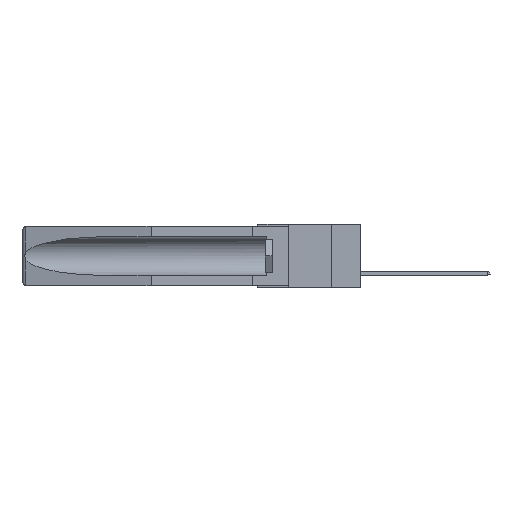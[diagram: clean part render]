
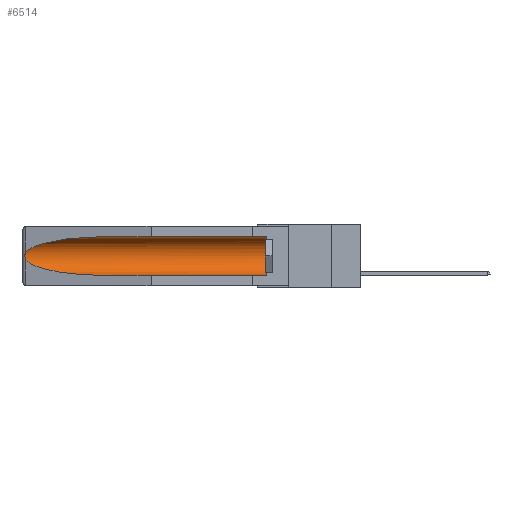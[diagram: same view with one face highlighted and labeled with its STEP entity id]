
A CAD part, left-side view. The second image highlights one B-rep face of the part: STEP entity #6514.
In plain terms, the highlighted cylindrical face has radius 2.857 mm (diameter 5.715 mm), a partial arc.
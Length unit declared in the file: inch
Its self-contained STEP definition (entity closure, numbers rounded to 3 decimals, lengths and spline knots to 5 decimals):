
#280 = CARTESIAN_POINT ( 'NONE',  ( 0.155, -0.30754, -0.1715 ) ) ;
#598 = CARTESIAN_POINT ( 'NONE',  ( 0.26537, 1.52718, -0.14972 ) ) ;
#786 = CARTESIAN_POINT ( 'NONE',  ( 0.155, 1.07973, -0.059 ) ) ;
#916 = ORIENTED_EDGE ( 'NONE', *, *, #7223, .T. ) ;
#985 = VERTEX_POINT ( 'NONE', #13216 ) ;
#1400 = VERTEX_POINT ( 'NONE', #3922 ) ;
#1910 = EDGE_CURVE ( 'NONE', #15032, #1400, #6840, .T. ) ;
#2029 = CARTESIAN_POINT ( 'NONE',  ( 0.2673, 1.5327, -0.16383 ) ) ;
#2625 = CARTESIAN_POINT ( 'NONE',  ( 0.155, 1.07973, -0.059 ) ) ;
#3262 = CARTESIAN_POINT ( 'NONE',  ( 0.26537, 1.52718, -0.19328 ) ) ;
#3442 = CARTESIAN_POINT ( 'NONE',  ( 0.26597, 1.52961, -0.15275 ) ) ;
#3922 = CARTESIAN_POINT ( 'NONE',  ( 0.26537, 1.52718, -0.19328 ) ) ;
#4167 = EDGE_CURVE ( 'NONE', #17128, #8973, #11744, .T. ) ;
#5041 = CARTESIAN_POINT ( 'NONE',  ( 0.155, 0.126, -0.284 ) ) ;
#5100 = EDGE_LOOP ( 'NONE', ( #5375, #6243, #15499, #18065, #916, #15361 ) ) ;
#5111 = EDGE_CURVE ( 'NONE', #8973, #15032, #5616, .T. ) ;
#5375 = ORIENTED_EDGE ( 'NONE', *, *, #5111, .T. ) ;
#5616 =( BOUNDED_CURVE ( )  B_SPLINE_CURVE ( 3, ( #786, #11089, #15373, #16802 ),
 .UNSPECIFIED., .F., .F. ) 
 B_SPLINE_CURVE_WITH_KNOTS ( ( 4, 4 ),
 ( 4.71239, 6.08839 ),
 .UNSPECIFIED. ) 
 CURVE ( )  GEOMETRIC_REPRESENTATION_ITEM ( )  RATIONAL_B_SPLINE_CURVE ( ( 1., 0.848, 0.848, 1. ) ) 
 REPRESENTATION_ITEM ( '' )  );
#6062 = DIRECTION ( 'NONE',  ( 0., 0., 1. ) ) ;
#6236 =( BOUNDED_CURVE ( )  B_SPLINE_CURVE ( 3, ( #3262, #13537, #9177, #13908 ),
 .UNSPECIFIED., .F., .F. ) 
 B_SPLINE_CURVE_WITH_KNOTS ( ( 4, 4 ),
 ( 0.1948, 1.5708 ),
 .UNSPECIFIED. ) 
 CURVE ( )  GEOMETRIC_REPRESENTATION_ITEM ( )  RATIONAL_B_SPLINE_CURVE ( ( 1., 0.848, 0.848, 1. ) ) 
 REPRESENTATION_ITEM ( '' )  );
#6243 = ORIENTED_EDGE ( 'NONE', *, *, #1910, .T. ) ;
#6263 = VERTEX_POINT ( 'NONE', #5041 ) ;
#6514 = ADVANCED_FACE ( 'NONE', ( #8643 ), #11636, .F. ) ;
#6644 = CARTESIAN_POINT ( 'NONE',  ( 0.26597, 1.5296, -0.19026 ) ) ;
#6840 = B_SPLINE_CURVE_WITH_KNOTS ( 'NONE', 3,
 ( #598, #3442, #9364, #2029, #12302, #13774, #10901, #18481, #6644, #12610 ),
 .UNSPECIFIED., .F., .F.,
 ( 4, 2, 2, 2, 4 ),
 ( 0., 0.00029, 0.00058, 0.00087, 0.00117 ),
 .UNSPECIFIED. ) ;
#6855 = DIRECTION ( 'NONE',  ( 0., -1., 0. ) ) ;
#7223 = EDGE_CURVE ( 'NONE', #6263, #17128, #14131, .T. ) ;
#8600 = AXIS2_PLACEMENT_3D ( 'NONE', #280, #14859, #6062 ) ;
#8643 = FACE_OUTER_BOUND ( 'NONE', #5100, .T. ) ;
#8701 = CARTESIAN_POINT ( 'NONE',  ( 0.155, -0.30754, -0.059 ) ) ;
#8755 = DIRECTION ( 'NONE',  ( 0., 1., 0. ) ) ;
#8973 = VERTEX_POINT ( 'NONE', #2625 ) ;
#9177 = CARTESIAN_POINT ( 'NONE',  ( 0.21114, 1.30732, -0.284 ) ) ;
#9364 = CARTESIAN_POINT ( 'NONE',  ( 0.26654, 1.53092, -0.15636 ) ) ;
#9549 = EDGE_CURVE ( 'NONE', #1400, #985, #6236, .T. ) ;
#10901 = CARTESIAN_POINT ( 'NONE',  ( 0.2673, 1.53269, -0.17917 ) ) ;
#11089 = CARTESIAN_POINT ( 'NONE',  ( 0.21114, 1.30732, -0.059 ) ) ;
#11636 = CYLINDRICAL_SURFACE ( 'NONE', #8600, 0.1125 ) ;
#11744 = LINE ( 'NONE', #8701, #17974 ) ;
#12199 = VECTOR ( 'NONE', #13444, 39.37008 ) ;
#12302 = CARTESIAN_POINT ( 'NONE',  ( 0.2675, 1.53308, -0.16763 ) ) ;
#12610 = CARTESIAN_POINT ( 'NONE',  ( 0.26537, 1.52718, -0.19328 ) ) ;
#13067 = EDGE_CURVE ( 'NONE', #6263, #985, #16788, .T. ) ;
#13182 = CARTESIAN_POINT ( 'NONE',  ( 0.155, -0.30754, -0.284 ) ) ;
#13216 = CARTESIAN_POINT ( 'NONE',  ( 0.155, 1.07973, -0.284 ) ) ;
#13444 = DIRECTION ( 'NONE',  ( 0., 1., 0. ) ) ;
#13537 = CARTESIAN_POINT ( 'NONE',  ( 0.25451, 1.48313, -0.24835 ) ) ;
#13774 = CARTESIAN_POINT ( 'NONE',  ( 0.2675, 1.53308, -0.17534 ) ) ;
#13908 = CARTESIAN_POINT ( 'NONE',  ( 0.155, 1.07973, -0.284 ) ) ;
#14131 = CIRCLE ( 'NONE', #14753, 0.1125 ) ;
#14228 = CARTESIAN_POINT ( 'NONE',  ( 0.155, 0.126, -0.059 ) ) ;
#14753 = AXIS2_PLACEMENT_3D ( 'NONE', #15658, #6855, #17199 ) ;
#14859 = DIRECTION ( 'NONE',  ( 0., 1., 0. ) ) ;
#15032 = VERTEX_POINT ( 'NONE', #15625 ) ;
#15361 = ORIENTED_EDGE ( 'NONE', *, *, #4167, .T. ) ;
#15373 = CARTESIAN_POINT ( 'NONE',  ( 0.25451, 1.48313, -0.09465 ) ) ;
#15499 = ORIENTED_EDGE ( 'NONE', *, *, #9549, .T. ) ;
#15625 = CARTESIAN_POINT ( 'NONE',  ( 0.26537, 1.52718, -0.14972 ) ) ;
#15658 = CARTESIAN_POINT ( 'NONE',  ( 0.155, 0.126, -0.1715 ) ) ;
#16788 = LINE ( 'NONE', #13182, #12199 ) ;
#16802 = CARTESIAN_POINT ( 'NONE',  ( 0.26537, 1.52718, -0.14972 ) ) ;
#17128 = VERTEX_POINT ( 'NONE', #14228 ) ;
#17199 = DIRECTION ( 'NONE',  ( 0., 0., 1. ) ) ;
#17974 = VECTOR ( 'NONE', #8755, 39.37008 ) ;
#18065 = ORIENTED_EDGE ( 'NONE', *, *, #13067, .F. ) ;
#18481 = CARTESIAN_POINT ( 'NONE',  ( 0.26655, 1.53094, -0.18657 ) ) ;
